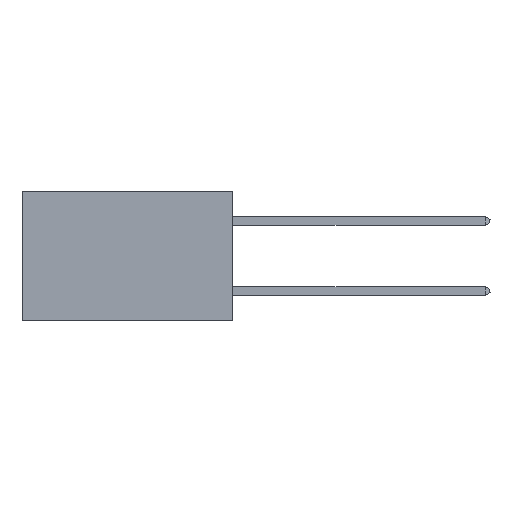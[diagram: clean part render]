
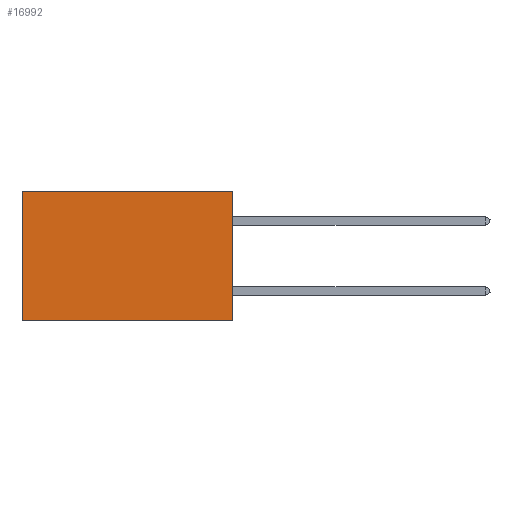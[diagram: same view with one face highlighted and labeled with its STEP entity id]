
A CAD part, left-side view. The second image highlights one B-rep face of the part: STEP entity #16992.
In plain terms, the highlighted planar face has unit normal (-1, 0, 0).
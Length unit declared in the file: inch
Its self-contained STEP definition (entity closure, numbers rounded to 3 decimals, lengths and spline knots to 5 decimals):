
#2627 = EDGE_CURVE ( 'NONE', #16653, #9622, #7370, .T. ) ;
#3554 = PLANE ( 'NONE',  #4511 ) ;
#3687 = VECTOR ( 'NONE', #12347, 39.37008 ) ;
#3899 = CARTESIAN_POINT ( 'NONE',  ( 0.2875, 0., -0.37 ) ) ;
#3955 = VECTOR ( 'NONE', #5956, 39.37008 ) ;
#4511 = AXIS2_PLACEMENT_3D ( 'NONE', #13913, #16457, #29463 ) ;
#5956 = DIRECTION ( 'NONE',  ( 0., 0., -1. ) ) ;
#6653 = ORIENTED_EDGE ( 'NONE', *, *, #30975, .F. ) ;
#7218 = EDGE_CURVE ( 'NONE', #16653, #33181, #21102, .T. ) ;
#7370 = LINE ( 'NONE', #8384, #24971 ) ;
#7437 = CARTESIAN_POINT ( 'NONE',  ( 0.2875, 0.6, 0. ) ) ;
#8357 = CARTESIAN_POINT ( 'NONE',  ( 0.2875, 0., 0. ) ) ;
#8384 = CARTESIAN_POINT ( 'NONE',  ( 0.2875, 0., 0. ) ) ;
#9622 = VERTEX_POINT ( 'NONE', #7437 ) ;
#11677 = FACE_OUTER_BOUND ( 'NONE', #12522, .T. ) ;
#12347 = DIRECTION ( 'NONE',  ( 0., 0., -1. ) ) ;
#12522 = EDGE_LOOP ( 'NONE', ( #25154, #6653, #24638, #21592 ) ) ;
#13913 = CARTESIAN_POINT ( 'NONE',  ( 0.2875, 0., 0. ) ) ;
#16457 = DIRECTION ( 'NONE',  ( 1., 0., 0. ) ) ;
#16653 = VERTEX_POINT ( 'NONE', #20432 ) ;
#16992 = ADVANCED_FACE ( 'NONE', ( #11677 ), #3554, .F. ) ;
#17352 = CARTESIAN_POINT ( 'NONE',  ( 0.2875, 0.6, -0.37 ) ) ;
#18287 = EDGE_CURVE ( 'NONE', #9622, #33103, #21227, .T. ) ;
#18643 = DIRECTION ( 'NONE',  ( 0., 1., 0. ) ) ;
#20432 = CARTESIAN_POINT ( 'NONE',  ( 0.2875, 0., 0. ) ) ;
#21102 = LINE ( 'NONE', #8357, #3955 ) ;
#21227 = LINE ( 'NONE', #25196, #3687 ) ;
#21592 = ORIENTED_EDGE ( 'NONE', *, *, #2627, .T. ) ;
#21833 = LINE ( 'NONE', #3899, #28001 ) ;
#24638 = ORIENTED_EDGE ( 'NONE', *, *, #7218, .F. ) ;
#24971 = VECTOR ( 'NONE', #18643, 39.37008 ) ;
#25154 = ORIENTED_EDGE ( 'NONE', *, *, #18287, .T. ) ;
#25196 = CARTESIAN_POINT ( 'NONE',  ( 0.2875, 0.6, 0. ) ) ;
#26904 = DIRECTION ( 'NONE',  ( 0., 1., 0. ) ) ;
#28001 = VECTOR ( 'NONE', #26904, 39.37008 ) ;
#28110 = CARTESIAN_POINT ( 'NONE',  ( 0.2875, 0., -0.37 ) ) ;
#29463 = DIRECTION ( 'NONE',  ( 0., 0., -1. ) ) ;
#30975 = EDGE_CURVE ( 'NONE', #33181, #33103, #21833, .T. ) ;
#33103 = VERTEX_POINT ( 'NONE', #17352 ) ;
#33181 = VERTEX_POINT ( 'NONE', #28110 ) ;
